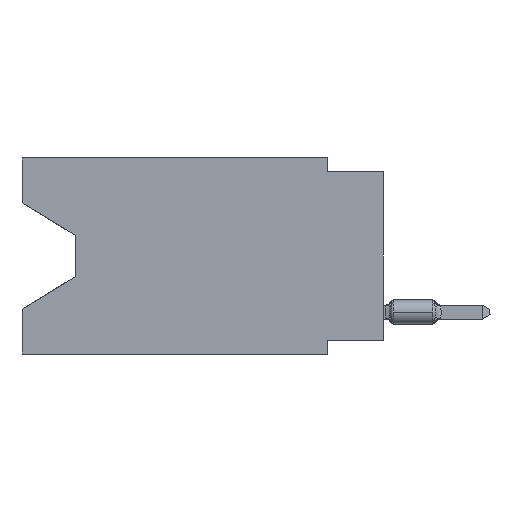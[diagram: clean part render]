
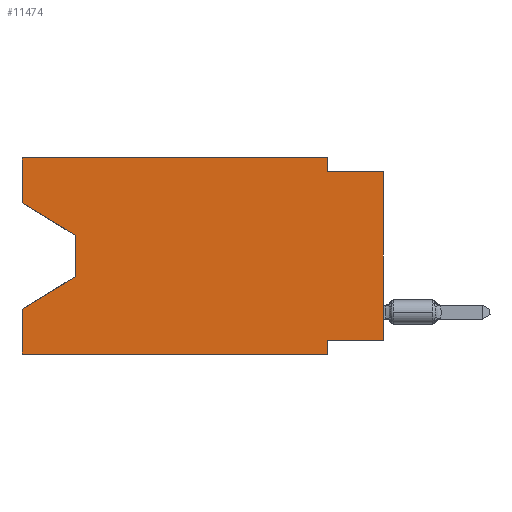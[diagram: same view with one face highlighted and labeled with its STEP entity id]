
A CAD part, left-side view. The second image highlights one B-rep face of the part: STEP entity #11474.
In plain terms, the highlighted planar face has unit normal (-1, 0, 0).
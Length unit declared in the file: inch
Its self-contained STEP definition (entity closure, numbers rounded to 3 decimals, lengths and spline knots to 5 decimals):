
#409 = CARTESIAN_POINT ( 'NONE',  ( 0., 0.645, 0. ) ) ;
#858 = EDGE_CURVE ( 'NONE', #33161, #17733, #22385, .T. ) ;
#1179 = VECTOR ( 'NONE', #47859, 39.37008 ) ;
#2233 = DIRECTION ( 'NONE',  ( 0., 1., 0. ) ) ;
#2545 = EDGE_LOOP ( 'NONE', ( #16520, #44207, #27509, #47855, #41752, #14013, #48177, #21431, #8058, #41868, #34510, #12081 ) ) ;
#2650 = AXIS2_PLACEMENT_3D ( 'NONE', #409, #49677, #42170 ) ;
#2728 = VECTOR ( 'NONE', #34582, 39.37008 ) ;
#2939 = LINE ( 'NONE', #45412, #41083 ) ;
#3261 = VECTOR ( 'NONE', #2233, 39.37008 ) ;
#4261 = DIRECTION ( 'NONE',  ( 0., 0., -1. ) ) ;
#5260 = LINE ( 'NONE', #12062, #18035 ) ;
#5332 = DIRECTION ( 'NONE',  ( 0., -0.855, -0.519 ) ) ;
#7185 = CARTESIAN_POINT ( 'NONE',  ( 0., 0.1, -0.35 ) ) ;
#7386 = CARTESIAN_POINT ( 'NONE',  ( 0., 0.645, -0.35 ) ) ;
#8058 = ORIENTED_EDGE ( 'NONE', *, *, #29945, .F. ) ;
#10169 = CARTESIAN_POINT ( 'NONE',  ( 0., 0., 0. ) ) ;
#10218 = CARTESIAN_POINT ( 'NONE',  ( 0., 0.1, -0.025 ) ) ;
#11251 = DIRECTION ( 'NONE',  ( 0., 0., -1. ) ) ;
#11474 = ADVANCED_FACE ( 'NONE', ( #34642 ), #15509, .F. ) ;
#11595 = DIRECTION ( 'NONE',  ( 0., 0., 1. ) ) ;
#11671 = VERTEX_POINT ( 'NONE', #29507 ) ;
#11703 = CARTESIAN_POINT ( 'NONE',  ( 0., 0.55, -0.212 ) ) ;
#11905 = VECTOR ( 'NONE', #31840, 39.37008 ) ;
#12062 = CARTESIAN_POINT ( 'NONE',  ( 0., 0.1, -0.35 ) ) ;
#12081 = ORIENTED_EDGE ( 'NONE', *, *, #46315, .F. ) ;
#12684 = CARTESIAN_POINT ( 'NONE',  ( 0., 0.645, 0. ) ) ;
#13308 = EDGE_CURVE ( 'NONE', #19144, #18907, #21718, .T. ) ;
#13930 = VECTOR ( 'NONE', #28776, 39.37008 ) ;
#14013 = ORIENTED_EDGE ( 'NONE', *, *, #24518, .F. ) ;
#14623 = LINE ( 'NONE', #30972, #26678 ) ;
#15509 = PLANE ( 'NONE',  #2650 ) ;
#15739 = EDGE_CURVE ( 'NONE', #33161, #32485, #33733, .T. ) ;
#16444 = CARTESIAN_POINT ( 'NONE',  ( 0., 0.55, -0.138 ) ) ;
#16520 = ORIENTED_EDGE ( 'NONE', *, *, #37268, .T. ) ;
#17733 = VERTEX_POINT ( 'NONE', #7185 ) ;
#17814 = LINE ( 'NONE', #33184, #30549 ) ;
#18035 = VECTOR ( 'NONE', #4261, 39.37008 ) ;
#18468 = CARTESIAN_POINT ( 'NONE',  ( 0., 0., -0.025 ) ) ;
#18907 = VERTEX_POINT ( 'NONE', #18468 ) ;
#19144 = VERTEX_POINT ( 'NONE', #20958 ) ;
#19500 = LINE ( 'NONE', #27052, #11905 ) ;
#20900 = CARTESIAN_POINT ( 'NONE',  ( 0., 0.55, -0.212 ) ) ;
#20958 = CARTESIAN_POINT ( 'NONE',  ( 0., 0., -0.325 ) ) ;
#21431 = ORIENTED_EDGE ( 'NONE', *, *, #13308, .T. ) ;
#21718 = LINE ( 'NONE', #10169, #1179 ) ;
#22385 = LINE ( 'NONE', #26899, #33490 ) ;
#23346 = VERTEX_POINT ( 'NONE', #39878 ) ;
#24280 = VERTEX_POINT ( 'NONE', #32748 ) ;
#24518 = EDGE_CURVE ( 'NONE', #23346, #17733, #5260, .T. ) ;
#26423 = CARTESIAN_POINT ( 'NONE',  ( 0., 0.645, 0. ) ) ;
#26678 = VECTOR ( 'NONE', #39223, 39.37008 ) ;
#26899 = CARTESIAN_POINT ( 'NONE',  ( 0., 0.645, -0.35 ) ) ;
#27052 = CARTESIAN_POINT ( 'NONE',  ( 0., 0., -0.025 ) ) ;
#27509 = ORIENTED_EDGE ( 'NONE', *, *, #34277, .T. ) ;
#27512 = LINE ( 'NONE', #11703, #2728 ) ;
#28776 = DIRECTION ( 'NONE',  ( 0., -1., 0. ) ) ;
#29507 = CARTESIAN_POINT ( 'NONE',  ( 0., 0.1, 0. ) ) ;
#29945 = EDGE_CURVE ( 'NONE', #41076, #18907, #19500, .T. ) ;
#30381 = VECTOR ( 'NONE', #11595, 39.37008 ) ;
#30549 = VECTOR ( 'NONE', #40945, 39.37008 ) ;
#30972 = CARTESIAN_POINT ( 'NONE',  ( 0., 0.55, -0.138 ) ) ;
#31840 = DIRECTION ( 'NONE',  ( 0., -1., 0. ) ) ;
#32051 = LINE ( 'NONE', #12684, #13930 ) ;
#32232 = CARTESIAN_POINT ( 'NONE',  ( 0., 0.645, -0.08025 ) ) ;
#32345 = VECTOR ( 'NONE', #5332, 39.37008 ) ;
#32485 = VERTEX_POINT ( 'NONE', #47937 ) ;
#32748 = CARTESIAN_POINT ( 'NONE',  ( 0., 0.645, 0. ) ) ;
#33161 = VERTEX_POINT ( 'NONE', #7386 ) ;
#33184 = CARTESIAN_POINT ( 'NONE',  ( 0., 0.645, 0. ) ) ;
#33490 = VECTOR ( 'NONE', #42222, 39.37008 ) ;
#33733 = LINE ( 'NONE', #26423, #30381 ) ;
#34277 = EDGE_CURVE ( 'NONE', #40088, #32485, #27512, .T. ) ;
#34482 = VERTEX_POINT ( 'NONE', #16444 ) ;
#34510 = ORIENTED_EDGE ( 'NONE', *, *, #41252, .F. ) ;
#34582 = DIRECTION ( 'NONE',  ( 0., 0.855, -0.519 ) ) ;
#34642 = FACE_OUTER_BOUND ( 'NONE', #2545, .T. ) ;
#35951 = CARTESIAN_POINT ( 'NONE',  ( 0., 0., -0.325 ) ) ;
#37268 = EDGE_CURVE ( 'NONE', #38966, #34482, #48052, .T. ) ;
#37529 = EDGE_CURVE ( 'NONE', #34482, #40088, #14623, .T. ) ;
#38966 = VERTEX_POINT ( 'NONE', #32232 ) ;
#39223 = DIRECTION ( 'NONE',  ( 0., 0., -1. ) ) ;
#39878 = CARTESIAN_POINT ( 'NONE',  ( 0., 0.1, -0.325 ) ) ;
#40088 = VERTEX_POINT ( 'NONE', #20900 ) ;
#40537 = CARTESIAN_POINT ( 'NONE',  ( 0., 0.645, -0.08025 ) ) ;
#40945 = DIRECTION ( 'NONE',  ( 0., 0., 1. ) ) ;
#41076 = VERTEX_POINT ( 'NONE', #10218 ) ;
#41083 = VECTOR ( 'NONE', #11251, 39.37008 ) ;
#41252 = EDGE_CURVE ( 'NONE', #24280, #11671, #32051, .T. ) ;
#41752 = ORIENTED_EDGE ( 'NONE', *, *, #858, .T. ) ;
#41868 = ORIENTED_EDGE ( 'NONE', *, *, #49192, .F. ) ;
#42170 = DIRECTION ( 'NONE',  ( 0., 0., -1. ) ) ;
#42222 = DIRECTION ( 'NONE',  ( 0., -1., 0. ) ) ;
#44207 = ORIENTED_EDGE ( 'NONE', *, *, #37529, .T. ) ;
#45412 = CARTESIAN_POINT ( 'NONE',  ( 0., 0.1, 0. ) ) ;
#46217 = EDGE_CURVE ( 'NONE', #19144, #23346, #48472, .T. ) ;
#46315 = EDGE_CURVE ( 'NONE', #38966, #24280, #17814, .T. ) ;
#47855 = ORIENTED_EDGE ( 'NONE', *, *, #15739, .F. ) ;
#47859 = DIRECTION ( 'NONE',  ( 0., 0., 1. ) ) ;
#47937 = CARTESIAN_POINT ( 'NONE',  ( 0., 0.645, -0.26975 ) ) ;
#48052 = LINE ( 'NONE', #40537, #32345 ) ;
#48177 = ORIENTED_EDGE ( 'NONE', *, *, #46217, .F. ) ;
#48472 = LINE ( 'NONE', #35951, #3261 ) ;
#49192 = EDGE_CURVE ( 'NONE', #11671, #41076, #2939, .T. ) ;
#49677 = DIRECTION ( 'NONE',  ( 1., 0., 0. ) ) ;
